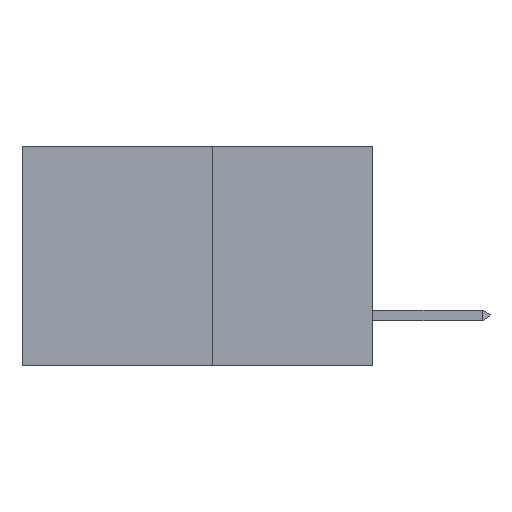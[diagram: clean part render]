
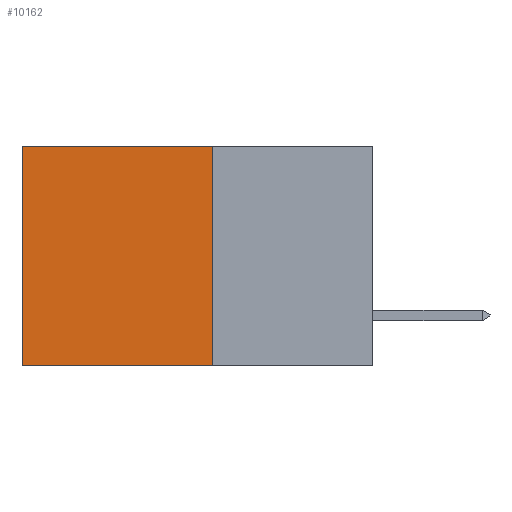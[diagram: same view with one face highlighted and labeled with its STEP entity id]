
A CAD part, left-side view. The second image highlights one B-rep face of the part: STEP entity #10162.
In plain terms, the highlighted planar face has unit normal (-1, 0, 0).
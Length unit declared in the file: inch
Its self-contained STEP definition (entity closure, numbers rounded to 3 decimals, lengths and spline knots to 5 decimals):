
#164 = LINE ( 'NONE', #8000, #4053 ) ;
#1010 = CARTESIAN_POINT ( 'NONE',  ( 0.277, 0.27, 0. ) ) ;
#1052 = EDGE_CURVE ( 'NONE', #11742, #12767, #164, .T. ) ;
#2053 = EDGE_CURVE ( 'NONE', #5586, #11742, #11231, .T. ) ;
#2211 = DIRECTION ( 'NONE',  ( 0., 0., -1. ) ) ;
#2482 = VECTOR ( 'NONE', #5722, 39.37008 ) ;
#2661 = ORIENTED_EDGE ( 'NONE', *, *, #7194, .T. ) ;
#2789 = LINE ( 'NONE', #6672, #2482 ) ;
#2937 = CARTESIAN_POINT ( 'NONE',  ( 0.277, 0.59, -0.37 ) ) ;
#3075 = CARTESIAN_POINT ( 'NONE',  ( 0.277, 0.59, 0. ) ) ;
#3285 = DIRECTION ( 'NONE',  ( 0., 1., 0. ) ) ;
#3561 = ORIENTED_EDGE ( 'NONE', *, *, #1052, .F. ) ;
#4053 = VECTOR ( 'NONE', #3285, 39.37008 ) ;
#4146 = CARTESIAN_POINT ( 'NONE',  ( 0.277, 0.27, -0.37 ) ) ;
#4858 = CARTESIAN_POINT ( 'NONE',  ( 0.277, 0.27, -0.37 ) ) ;
#5586 = VERTEX_POINT ( 'NONE', #1010 ) ;
#5722 = DIRECTION ( 'NONE',  ( 0., 1., 0. ) ) ;
#5771 = ORIENTED_EDGE ( 'NONE', *, *, #2053, .F. ) ;
#6563 = CARTESIAN_POINT ( 'NONE',  ( 0.277, 0.59, -0.37 ) ) ;
#6672 = CARTESIAN_POINT ( 'NONE',  ( 0.277, 0.27, 0. ) ) ;
#6869 = FACE_OUTER_BOUND ( 'NONE', #7839, .T. ) ;
#6901 = VECTOR ( 'NONE', #8552, 39.37008 ) ;
#7145 = PLANE ( 'NONE',  #7938 ) ;
#7194 = EDGE_CURVE ( 'NONE', #10771, #12767, #9528, .T. ) ;
#7635 = ORIENTED_EDGE ( 'NONE', *, *, #12228, .T. ) ;
#7839 = EDGE_LOOP ( 'NONE', ( #2661, #3561, #5771, #7635 ) ) ;
#7842 = CARTESIAN_POINT ( 'NONE',  ( 0.277, 0.27, -0.37 ) ) ;
#7938 = AXIS2_PLACEMENT_3D ( 'NONE', #4146, #8124, #2211 ) ;
#8000 = CARTESIAN_POINT ( 'NONE',  ( 0.277, 0.27, -0.37 ) ) ;
#8124 = DIRECTION ( 'NONE',  ( 1., 0., 0. ) ) ;
#8240 = VECTOR ( 'NONE', #8944, 39.37008 ) ;
#8552 = DIRECTION ( 'NONE',  ( 0., 0., -1. ) ) ;
#8944 = DIRECTION ( 'NONE',  ( 0., 0., -1. ) ) ;
#9528 = LINE ( 'NONE', #6563, #6901 ) ;
#10162 = ADVANCED_FACE ( 'NONE', ( #6869 ), #7145, .F. ) ;
#10771 = VERTEX_POINT ( 'NONE', #3075 ) ;
#11231 = LINE ( 'NONE', #7842, #8240 ) ;
#11742 = VERTEX_POINT ( 'NONE', #4858 ) ;
#12228 = EDGE_CURVE ( 'NONE', #5586, #10771, #2789, .T. ) ;
#12767 = VERTEX_POINT ( 'NONE', #2937 ) ;
